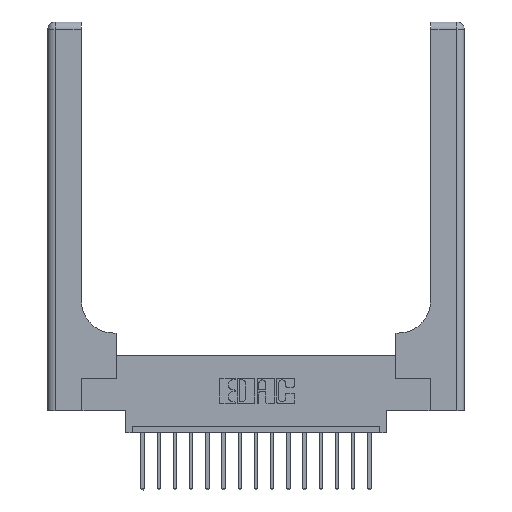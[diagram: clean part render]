
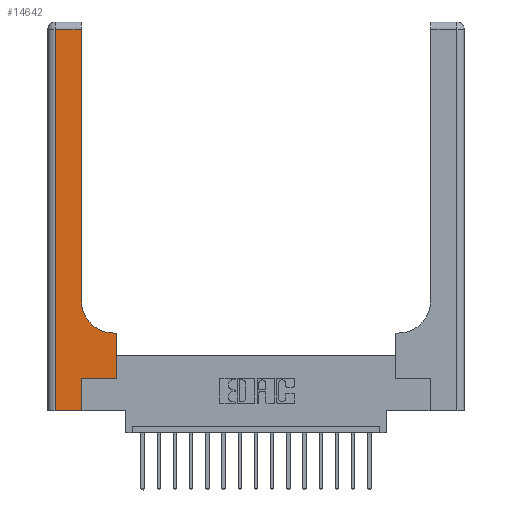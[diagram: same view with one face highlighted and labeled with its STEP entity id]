
A CAD part, top view. The second image highlights one B-rep face of the part: STEP entity #14642.
In plain terms, the highlighted planar face has unit normal (0, 0, 1).
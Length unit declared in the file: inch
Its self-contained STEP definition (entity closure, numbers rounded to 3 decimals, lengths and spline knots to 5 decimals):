
#460 = DIRECTION ( 'NONE',  ( 0., 0., -1. ) ) ;
#1378 = EDGE_CURVE ( 'NONE', #17423, #17868, #13720, .T. ) ;
#1484 = FACE_OUTER_BOUND ( 'NONE', #2350, .T. ) ;
#1986 = VERTEX_POINT ( 'NONE', #6327 ) ;
#2045 = LINE ( 'NONE', #7852, #9101 ) ;
#2161 = VECTOR ( 'NONE', #7267, 39.37008 ) ;
#2350 = EDGE_LOOP ( 'NONE', ( #3848, #5233, #2917, #3613, #8595, #8887, #14717, #16453, #3563 ) ) ;
#2390 = LINE ( 'NONE', #11135, #16093 ) ;
#2525 = DIRECTION ( 'NONE',  ( 1., 0., 0. ) ) ;
#2917 = ORIENTED_EDGE ( 'NONE', *, *, #12105, .T. ) ;
#3000 = VECTOR ( 'NONE', #9694, 39.37008 ) ;
#3104 = CARTESIAN_POINT ( 'NONE',  ( 0.528, 0.25, 0.37 ) ) ;
#3274 = EDGE_CURVE ( 'NONE', #10060, #1986, #2045, .T. ) ;
#3356 = EDGE_CURVE ( 'NONE', #17868, #8430, #15159, .T. ) ;
#3549 = CARTESIAN_POINT ( 'NONE',  ( 0.06, 0., 0.37 ) ) ;
#3563 = ORIENTED_EDGE ( 'NONE', *, *, #1378, .T. ) ;
#3568 = EDGE_CURVE ( 'NONE', #4257, #10060, #14703, .T. ) ;
#3613 = ORIENTED_EDGE ( 'NONE', *, *, #8363, .T. ) ;
#3751 = VERTEX_POINT ( 'NONE', #17186 ) ;
#3848 = ORIENTED_EDGE ( 'NONE', *, *, #3356, .T. ) ;
#4257 = VERTEX_POINT ( 'NONE', #7437 ) ;
#4634 = CARTESIAN_POINT ( 'NONE',  ( 0., 3., 0.37 ) ) ;
#5233 = ORIENTED_EDGE ( 'NONE', *, *, #5917, .T. ) ;
#5290 = LINE ( 'NONE', #9627, #2161 ) ;
#5598 = LINE ( 'NONE', #3104, #6030 ) ;
#5917 = EDGE_CURVE ( 'NONE', #8430, #12894, #15332, .T. ) ;
#6016 = VECTOR ( 'NONE', #8228, 39.37008 ) ;
#6030 = VECTOR ( 'NONE', #12969, 39.37008 ) ;
#6059 = DIRECTION ( 'NONE',  ( -1., 0., 0. ) ) ;
#6132 = AXIS2_PLACEMENT_3D ( 'NONE', #10137, #15920, #6144 ) ;
#6144 = DIRECTION ( 'NONE',  ( 1., 0., 0. ) ) ;
#6327 = CARTESIAN_POINT ( 'NONE',  ( 0.528, 0.25, 0.37 ) ) ;
#7267 = DIRECTION ( 'NONE',  ( -1., 0., 0. ) ) ;
#7286 = DIRECTION ( 'NONE',  ( 0., -1., 0. ) ) ;
#7437 = CARTESIAN_POINT ( 'NONE',  ( 0.265, 0., 0.37 ) ) ;
#7852 = CARTESIAN_POINT ( 'NONE',  ( 0.265, 0.25, 0.37 ) ) ;
#8006 = CARTESIAN_POINT ( 'NONE',  ( 0.265, 0.25, 0.37 ) ) ;
#8173 = CARTESIAN_POINT ( 'NONE',  ( 0., 2.94, 0.37 ) ) ;
#8228 = DIRECTION ( 'NONE',  ( -1., 0., 0. ) ) ;
#8363 = EDGE_CURVE ( 'NONE', #9443, #4257, #2390, .T. ) ;
#8430 = VERTEX_POINT ( 'NONE', #16803 ) ;
#8595 = ORIENTED_EDGE ( 'NONE', *, *, #3568, .T. ) ;
#8662 = CARTESIAN_POINT ( 'NONE',  ( 0.26, 0.85, 0.37 ) ) ;
#8887 = ORIENTED_EDGE ( 'NONE', *, *, #3274, .T. ) ;
#9101 = VECTOR ( 'NONE', #10588, 39.37008 ) ;
#9443 = VERTEX_POINT ( 'NONE', #3549 ) ;
#9627 = CARTESIAN_POINT ( 'NONE',  ( 0.26, 0.6, 0.37 ) ) ;
#9694 = DIRECTION ( 'NONE',  ( 0., 1., 0. ) ) ;
#9713 = CARTESIAN_POINT ( 'NONE',  ( 0.06, 2.94, 0.37 ) ) ;
#9930 = CARTESIAN_POINT ( 'NONE',  ( 0.06, 3., 0.37 ) ) ;
#10060 = VERTEX_POINT ( 'NONE', #8006 ) ;
#10137 = CARTESIAN_POINT ( 'NONE',  ( 0.51, 0.85, 0.37 ) ) ;
#10588 = DIRECTION ( 'NONE',  ( 1., 0., 0. ) ) ;
#11135 = CARTESIAN_POINT ( 'NONE',  ( 0., 0., 0.37 ) ) ;
#11359 = VECTOR ( 'NONE', #15117, 39.37008 ) ;
#12105 = EDGE_CURVE ( 'NONE', #12894, #9443, #15273, .T. ) ;
#12894 = VERTEX_POINT ( 'NONE', #9713 ) ;
#12969 = DIRECTION ( 'NONE',  ( 0., 1., 0. ) ) ;
#13194 = EDGE_CURVE ( 'NONE', #3751, #17423, #5290, .T. ) ;
#13720 = CIRCLE ( 'NONE', #6132, 0.25 ) ;
#13969 = CARTESIAN_POINT ( 'NONE',  ( 0.265, 0., 0.37 ) ) ;
#14191 = AXIS2_PLACEMENT_3D ( 'NONE', #4634, #460, #6059 ) ;
#14642 = ADVANCED_FACE ( 'NONE', ( #1484 ), #15949, .F. ) ;
#14703 = LINE ( 'NONE', #13969, #3000 ) ;
#14717 = ORIENTED_EDGE ( 'NONE', *, *, #16842, .T. ) ;
#14808 = VECTOR ( 'NONE', #7286, 39.37008 ) ;
#15117 = DIRECTION ( 'NONE',  ( 0., 1., 0. ) ) ;
#15159 = LINE ( 'NONE', #15244, #11359 ) ;
#15244 = CARTESIAN_POINT ( 'NONE',  ( 0.26, 3., 0.37 ) ) ;
#15273 = LINE ( 'NONE', #9930, #14808 ) ;
#15332 = LINE ( 'NONE', #8173, #6016 ) ;
#15920 = DIRECTION ( 'NONE',  ( 0., 0., -1. ) ) ;
#15949 = PLANE ( 'NONE',  #14191 ) ;
#16093 = VECTOR ( 'NONE', #2525, 39.37008 ) ;
#16147 = CARTESIAN_POINT ( 'NONE',  ( 0.51, 0.6, 0.37 ) ) ;
#16453 = ORIENTED_EDGE ( 'NONE', *, *, #13194, .T. ) ;
#16803 = CARTESIAN_POINT ( 'NONE',  ( 0.26, 2.94, 0.37 ) ) ;
#16842 = EDGE_CURVE ( 'NONE', #1986, #3751, #5598, .T. ) ;
#17186 = CARTESIAN_POINT ( 'NONE',  ( 0.528, 0.6, 0.37 ) ) ;
#17423 = VERTEX_POINT ( 'NONE', #16147 ) ;
#17868 = VERTEX_POINT ( 'NONE', #8662 ) ;
